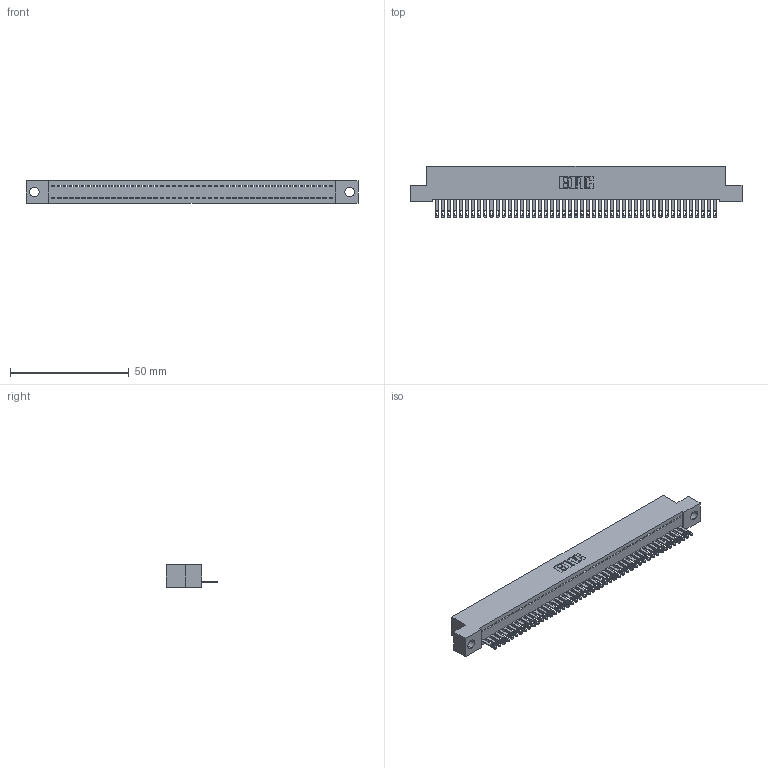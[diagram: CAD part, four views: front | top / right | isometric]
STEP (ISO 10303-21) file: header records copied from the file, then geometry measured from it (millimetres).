
FILE_DESCRIPTION (( 'STEP AP203' ), '1' );
FILE_NAME ('342-047-500-104.STEP', '2019-10-02T21:06:59', ( '' ), ( '' ), 'SwSTEP 2.0', 'SolidWorks 2016', '' );
FILE_SCHEMA (( 'CONFIG_CONTROL_DESIGN' ));
Length unit declared in the file: inch
Products named in the file (3): 342 Part_.156 TH; 345-292-001_345-293-100; 342-047-500-104
Assembly tree (48 placements, depth 2):
  342-047-500-104
    342 Part_.156 TH
    345-292-001_345-293-100  x47
Bounding box: 139.7 x 21.85 x 9.4 mm (x, y, z)
Volume: 12209.4 mm3; surface area: 17933.6 mm2
Topology: 48 solids, 48 shells, 2648 faces, 8195 edges, 5462 vertices
Faces by surface type: plane 1758, cylinder 890
Entity records: 27887 total; most frequent: CARTESIAN_POINT 4815, ORIENTED_EDGE 4798, DIRECTION 4053, EDGE_CURVE 2399, LINE 2267, VECTOR 2267, VERTEX_POINT 1598, AXIS2_PLACEMENT_3D 893
